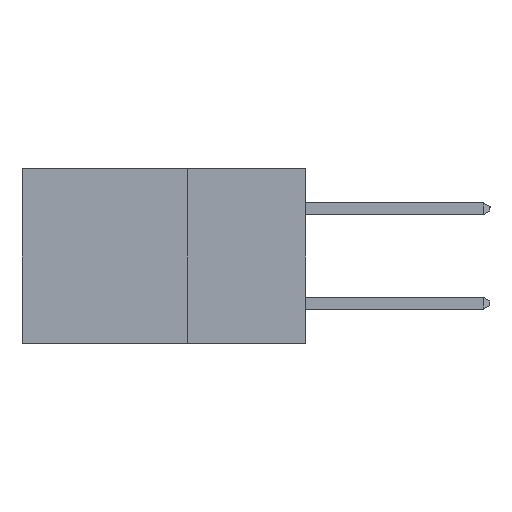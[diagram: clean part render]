
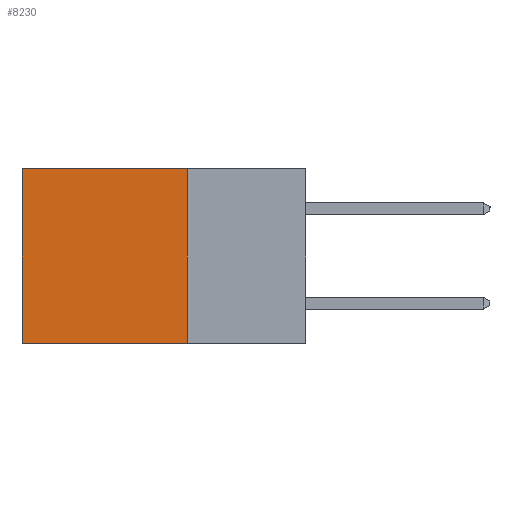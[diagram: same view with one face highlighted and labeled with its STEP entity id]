
A CAD part, left-side view. The second image highlights one B-rep face of the part: STEP entity #8230.
In plain terms, the highlighted planar face has unit normal (-1, 0, 0).
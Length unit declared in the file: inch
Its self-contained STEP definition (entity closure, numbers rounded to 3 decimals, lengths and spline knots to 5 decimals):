
#278 = LINE ( 'NONE', #9863, #7791 ) ;
#406 = CARTESIAN_POINT ( 'NONE',  ( 0.2615, 0.6, 0. ) ) ;
#670 = CARTESIAN_POINT ( 'NONE',  ( 0.2615, 0.25, -0.37 ) ) ;
#1289 = EDGE_CURVE ( 'NONE', #2766, #8249, #278, .T. ) ;
#1401 = CARTESIAN_POINT ( 'NONE',  ( 0.2615, 0.25, 0. ) ) ;
#1878 = DIRECTION ( 'NONE',  ( 0., 0., -1. ) ) ;
#2559 = VECTOR ( 'NONE', #6625, 39.37008 ) ;
#2766 = VERTEX_POINT ( 'NONE', #6306 ) ;
#2916 = VECTOR ( 'NONE', #8043, 39.37008 ) ;
#3494 = DIRECTION ( 'NONE',  ( 0., 1., 0. ) ) ;
#3970 = CARTESIAN_POINT ( 'NONE',  ( 0.2615, 0.25, -0.37 ) ) ;
#4029 = FACE_OUTER_BOUND ( 'NONE', #7040, .T. ) ;
#4454 = ORIENTED_EDGE ( 'NONE', *, *, #8124, .T. ) ;
#4786 = CARTESIAN_POINT ( 'NONE',  ( 0.2615, 0.6, -0.37 ) ) ;
#4842 = LINE ( 'NONE', #1401, #2559 ) ;
#5395 = CARTESIAN_POINT ( 'NONE',  ( 0.2615, 0.25, -0.37 ) ) ;
#5560 = VECTOR ( 'NONE', #3494, 39.37008 ) ;
#5593 = LINE ( 'NONE', #4786, #2916 ) ;
#5662 = AXIS2_PLACEMENT_3D ( 'NONE', #670, #11009, #9235 ) ;
#5846 = VERTEX_POINT ( 'NONE', #406 ) ;
#6306 = CARTESIAN_POINT ( 'NONE',  ( 0.2615, 0.25, 0. ) ) ;
#6625 = DIRECTION ( 'NONE',  ( 0., 1., 0. ) ) ;
#6931 = EDGE_CURVE ( 'NONE', #2766, #5846, #4842, .T. ) ;
#7040 = EDGE_LOOP ( 'NONE', ( #4454, #10360, #10815, #9622 ) ) ;
#7105 = LINE ( 'NONE', #5395, #5560 ) ;
#7791 = VECTOR ( 'NONE', #1878, 39.37008 ) ;
#8043 = DIRECTION ( 'NONE',  ( 0., 0., -1. ) ) ;
#8124 = EDGE_CURVE ( 'NONE', #5846, #11247, #5593, .T. ) ;
#8230 = ADVANCED_FACE ( 'NONE', ( #4029 ), #10310, .F. ) ;
#8249 = VERTEX_POINT ( 'NONE', #3970 ) ;
#8742 = CARTESIAN_POINT ( 'NONE',  ( 0.2615, 0.6, -0.37 ) ) ;
#9014 = EDGE_CURVE ( 'NONE', #8249, #11247, #7105, .T. ) ;
#9235 = DIRECTION ( 'NONE',  ( 0., 0., -1. ) ) ;
#9622 = ORIENTED_EDGE ( 'NONE', *, *, #6931, .T. ) ;
#9863 = CARTESIAN_POINT ( 'NONE',  ( 0.2615, 0.25, -0.37 ) ) ;
#10310 = PLANE ( 'NONE',  #5662 ) ;
#10360 = ORIENTED_EDGE ( 'NONE', *, *, #9014, .F. ) ;
#10815 = ORIENTED_EDGE ( 'NONE', *, *, #1289, .F. ) ;
#11009 = DIRECTION ( 'NONE',  ( 1., 0., 0. ) ) ;
#11247 = VERTEX_POINT ( 'NONE', #8742 ) ;
